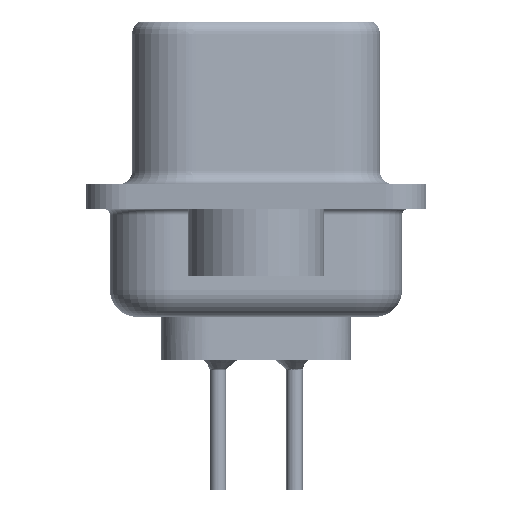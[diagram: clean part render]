
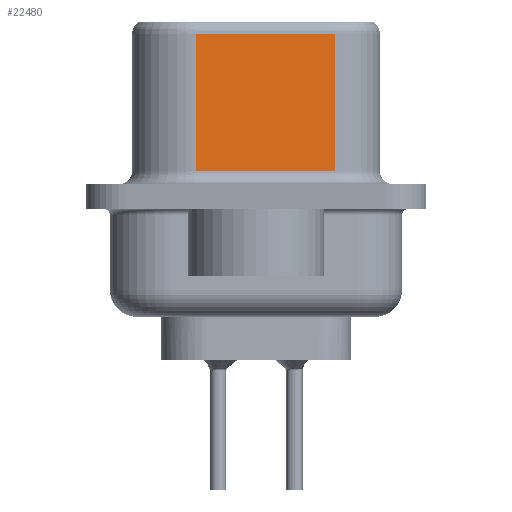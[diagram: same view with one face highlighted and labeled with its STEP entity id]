
A CAD part, left-side view. The second image highlights one B-rep face of the part: STEP entity #22480.
In plain terms, the highlighted planar face has unit normal (-0.985, -0.174, 0).
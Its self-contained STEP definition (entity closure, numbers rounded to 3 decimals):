
#798 = LINE ( 'NONE', #16905, #2669 ) ;
#1482 = LINE ( 'NONE', #26361, #5131 ) ;
#1590 = VERTEX_POINT ( 'NONE', #29175 ) ;
#2108 = VECTOR ( 'NONE', #24425, 1000. ) ;
#2669 = VECTOR ( 'NONE', #19423, 1000. ) ;
#4328 = AXIS2_PLACEMENT_3D ( 'NONE', #29312, #17710, #15477 ) ;
#4570 = VERTEX_POINT ( 'NONE', #28757 ) ;
#5131 = VECTOR ( 'NONE', #7614, 1000. ) ;
#7122 = ORIENTED_EDGE ( 'NONE', *, *, #12939, .F. ) ;
#7391 = EDGE_LOOP ( 'NONE', ( #7122, #24096, #10645, #23841 ) ) ;
#7614 = DIRECTION ( 'NONE',  ( 0., 0., -1. ) ) ;
#8614 = FACE_OUTER_BOUND ( 'NONE', #7391, .T. ) ;
#9271 = EDGE_CURVE ( 'NONE', #28448, #1590, #10732, .T. ) ;
#10645 = ORIENTED_EDGE ( 'NONE', *, *, #16004, .T. ) ;
#10732 = LINE ( 'NONE', #28739, #2108 ) ;
#11004 = EDGE_CURVE ( 'NONE', #20366, #4570, #798, .T. ) ;
#11771 = DIRECTION ( 'NONE',  ( 0., 0., -1. ) ) ;
#12939 = EDGE_CURVE ( 'NONE', #28448, #4570, #15652, .T. ) ;
#13426 = CARTESIAN_POINT ( 'NONE',  ( 4.58, -2.927, 6.52 ) ) ;
#15477 = DIRECTION ( 'NONE',  ( -0.174, 0.985, 0. ) ) ;
#15652 = LINE ( 'NONE', #13426, #25285 ) ;
#16004 = EDGE_CURVE ( 'NONE', #1590, #20366, #1482, .T. ) ;
#16034 = CARTESIAN_POINT ( 'NONE',  ( 4.58, -2.927, 6.02 ) ) ;
#16905 = CARTESIAN_POINT ( 'NONE',  ( 4.58, -2.927, 0.95 ) ) ;
#17710 = DIRECTION ( 'NONE',  ( 0.985, 0.174, 0. ) ) ;
#19423 = DIRECTION ( 'NONE',  ( 0.174, -0.985, 0. ) ) ;
#20366 = VERTEX_POINT ( 'NONE', #21338 ) ;
#21338 = CARTESIAN_POINT ( 'NONE',  ( 3.67, 2.233, 0.95 ) ) ;
#22461 = PLANE ( 'NONE',  #4328 ) ;
#22480 = ADVANCED_FACE ( 'NONE', ( #8614 ), #22461, .F. ) ;
#23841 = ORIENTED_EDGE ( 'NONE', *, *, #11004, .T. ) ;
#24096 = ORIENTED_EDGE ( 'NONE', *, *, #9271, .T. ) ;
#24425 = DIRECTION ( 'NONE',  ( -0.174, 0.985, 0. ) ) ;
#25285 = VECTOR ( 'NONE', #11771, 1000. ) ;
#26361 = CARTESIAN_POINT ( 'NONE',  ( 3.67, 2.233, 6.52 ) ) ;
#28448 = VERTEX_POINT ( 'NONE', #16034 ) ;
#28739 = CARTESIAN_POINT ( 'NONE',  ( 4.58, -2.927, 6.02 ) ) ;
#28757 = CARTESIAN_POINT ( 'NONE',  ( 4.58, -2.927, 0.95 ) ) ;
#29175 = CARTESIAN_POINT ( 'NONE',  ( 3.67, 2.233, 6.02 ) ) ;
#29312 = CARTESIAN_POINT ( 'NONE',  ( 4.58, -2.927, 6.52 ) ) ;
